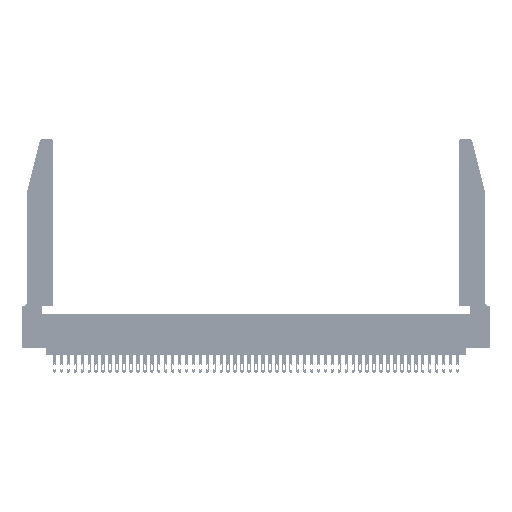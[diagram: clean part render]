
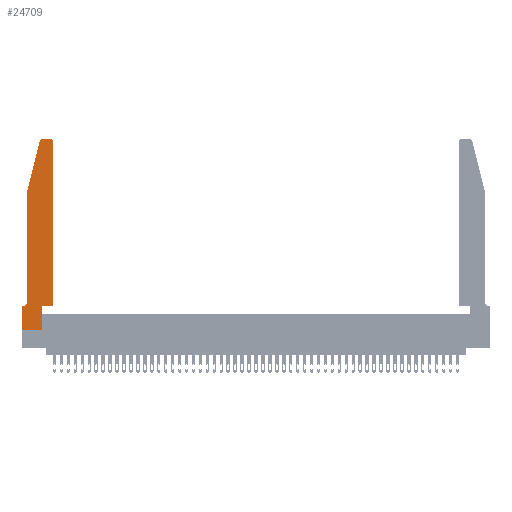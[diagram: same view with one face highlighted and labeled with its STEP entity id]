
A CAD part, top view. The second image highlights one B-rep face of the part: STEP entity #24709.
In plain terms, the highlighted planar face has unit normal (0, 0, 1).
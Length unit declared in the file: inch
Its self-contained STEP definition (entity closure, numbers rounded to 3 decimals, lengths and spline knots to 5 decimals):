
#183 = CIRCLE ( 'NONE', #768, 0.03 ) ;
#341 = DIRECTION ( 'NONE',  ( 0., 0., 1. ) ) ;
#351 = CARTESIAN_POINT ( 'NONE',  ( 0., 0.35, 0.37 ) ) ;
#488 = VECTOR ( 'NONE', #31601, 39.37008 ) ;
#573 = LINE ( 'NONE', #44899, #16606 ) ;
#768 = AXIS2_PLACEMENT_3D ( 'NONE', #4350, #11652, #34419 ) ;
#1428 = CARTESIAN_POINT ( 'NONE',  ( 0.2865, 0.35, 0.37 ) ) ;
#2223 = EDGE_CURVE ( 'NONE', #23543, #10127, #27594, .T. ) ;
#3217 = CARTESIAN_POINT ( 'NONE',  ( 0.2865, 0.35, 0.37 ) ) ;
#4350 = CARTESIAN_POINT ( 'NONE',  ( 0.4205, 2.72, 0.37 ) ) ;
#5069 = EDGE_CURVE ( 'NONE', #8838, #24708, #10907, .T. ) ;
#5454 = ORIENTED_EDGE ( 'NONE', *, *, #22700, .T. ) ;
#5991 = ORIENTED_EDGE ( 'NONE', *, *, #34411, .T. ) ;
#6038 = CARTESIAN_POINT ( 'NONE',  ( 0.4505, 0.35, 0.37 ) ) ;
#6975 = CARTESIAN_POINT ( 'NONE',  ( 0.4205, 2.75, 0.37 ) ) ;
#7641 = FACE_OUTER_BOUND ( 'NONE', #18019, .T. ) ;
#8130 = VERTEX_POINT ( 'NONE', #6975 ) ;
#8193 = LINE ( 'NONE', #1428, #44113 ) ;
#8483 = DIRECTION ( 'NONE',  ( -1., 0., 0. ) ) ;
#8838 = VERTEX_POINT ( 'NONE', #28938 ) ;
#9995 = DIRECTION ( 'NONE',  ( 1., 0., 0. ) ) ;
#10127 = VERTEX_POINT ( 'NONE', #24050 ) ;
#10395 = ORIENTED_EDGE ( 'NONE', *, *, #43474, .T. ) ;
#10548 = LINE ( 'NONE', #31767, #488 ) ;
#10907 = LINE ( 'NONE', #16419, #18087 ) ;
#10935 = ORIENTED_EDGE ( 'NONE', *, *, #39487, .T. ) ;
#10945 = VECTOR ( 'NONE', #14741, 39.37008 ) ;
#11652 = DIRECTION ( 'NONE',  ( 0., 0., 1. ) ) ;
#13085 = LINE ( 'NONE', #6038, #40780 ) ;
#13604 = AXIS2_PLACEMENT_3D ( 'NONE', #37990, #341, #46037 ) ;
#13871 = VERTEX_POINT ( 'NONE', #48773 ) ;
#14741 = DIRECTION ( 'NONE',  ( -1., 0., 0. ) ) ;
#14787 = EDGE_CURVE ( 'NONE', #31159, #8130, #183, .T. ) ;
#15461 = EDGE_CURVE ( 'NONE', #20353, #31159, #47329, .T. ) ;
#15609 = AXIS2_PLACEMENT_3D ( 'NONE', #18943, #45210, #19099 ) ;
#16419 = CARTESIAN_POINT ( 'NONE',  ( 0., 0., 0.37 ) ) ;
#16606 = VECTOR ( 'NONE', #29816, 39.37008 ) ;
#16960 = VERTEX_POINT ( 'NONE', #351 ) ;
#18019 = EDGE_LOOP ( 'NONE', ( #5991, #23481, #28074, #33410, #44886, #31744, #5454, #23098, #10395, #10935, #38307, #20407 ) ) ;
#18087 = VECTOR ( 'NONE', #31704, 39.37008 ) ;
#18943 = CARTESIAN_POINT ( 'NONE',  ( 0.284, 2.72, 0.37 ) ) ;
#19093 = CARTESIAN_POINT ( 'NONE',  ( 0.2865, 0., 0.37 ) ) ;
#19099 = DIRECTION ( 'NONE',  ( 1., 0., 0. ) ) ;
#19185 = VECTOR ( 'NONE', #32096, 39.37008 ) ;
#20084 = CARTESIAN_POINT ( 'NONE',  ( 0.0755, 2., 0.37 ) ) ;
#20353 = VERTEX_POINT ( 'NONE', #30305 ) ;
#20356 = LINE ( 'NONE', #20084, #19185 ) ;
#20407 = ORIENTED_EDGE ( 'NONE', *, *, #14787, .T. ) ;
#22700 = EDGE_CURVE ( 'NONE', #16960, #8838, #27076, .T. ) ;
#23098 = ORIENTED_EDGE ( 'NONE', *, *, #5069, .T. ) ;
#23361 = DIRECTION ( 'NONE',  ( 0., 0., -1. ) ) ;
#23481 = ORIENTED_EDGE ( 'NONE', *, *, #2223, .T. ) ;
#23543 = VERTEX_POINT ( 'NONE', #47120 ) ;
#23691 = CARTESIAN_POINT ( 'NONE',  ( 0.0055, 0.42, 0.37 ) ) ;
#24050 = CARTESIAN_POINT ( 'NONE',  ( 0.25487, 2.72718, 0.37 ) ) ;
#24708 = VERTEX_POINT ( 'NONE', #19093 ) ;
#24709 = ADVANCED_FACE ( 'NONE', ( #7641 ), #41604, .T. ) ;
#25517 = AXIS2_PLACEMENT_3D ( 'NONE', #23691, #23361, #8483 ) ;
#25555 = VERTEX_POINT ( 'NONE', #48331 ) ;
#25603 = VERTEX_POINT ( 'NONE', #26658 ) ;
#26585 = EDGE_CURVE ( 'NONE', #25603, #16960, #39849, .T. ) ;
#26658 = CARTESIAN_POINT ( 'NONE',  ( 0.0055, 0.35, 0.37 ) ) ;
#27047 = VERTEX_POINT ( 'NONE', #3217 ) ;
#27076 = LINE ( 'NONE', #34751, #48217 ) ;
#27254 = DIRECTION ( 'NONE',  ( 0., 1., 0. ) ) ;
#27514 = EDGE_CURVE ( 'NONE', #25555, #13871, #20356, .T. ) ;
#27594 = CIRCLE ( 'NONE', #15609, 0.03 ) ;
#28074 = ORIENTED_EDGE ( 'NONE', *, *, #37272, .T. ) ;
#28938 = CARTESIAN_POINT ( 'NONE',  ( 0., 0., 0.37 ) ) ;
#29816 = DIRECTION ( 'NONE',  ( -0.239, -0.971, 0. ) ) ;
#30305 = CARTESIAN_POINT ( 'NONE',  ( 0.4505, 0.35, 0.37 ) ) ;
#30716 = CIRCLE ( 'NONE', #25517, 0.07 ) ;
#31159 = VERTEX_POINT ( 'NONE', #36674 ) ;
#31601 = DIRECTION ( 'NONE',  ( -1., 0., 0. ) ) ;
#31704 = DIRECTION ( 'NONE',  ( 1., 0., 0. ) ) ;
#31744 = ORIENTED_EDGE ( 'NONE', *, *, #26585, .T. ) ;
#31767 = CARTESIAN_POINT ( 'NONE',  ( 0.2605, 2.75, 0.37 ) ) ;
#32096 = DIRECTION ( 'NONE',  ( 0., -1., 0. ) ) ;
#33410 = ORIENTED_EDGE ( 'NONE', *, *, #27514, .T. ) ;
#34261 = EDGE_CURVE ( 'NONE', #13871, #25603, #30716, .T. ) ;
#34411 = EDGE_CURVE ( 'NONE', #8130, #23543, #10548, .T. ) ;
#34419 = DIRECTION ( 'NONE',  ( 1., 0., 0. ) ) ;
#34751 = CARTESIAN_POINT ( 'NONE',  ( 0., 0., 0.37 ) ) ;
#36674 = CARTESIAN_POINT ( 'NONE',  ( 0.4505, 2.72, 0.37 ) ) ;
#37272 = EDGE_CURVE ( 'NONE', #10127, #25555, #573, .T. ) ;
#37598 = CARTESIAN_POINT ( 'NONE',  ( 0.0755, 0.35, 0.37 ) ) ;
#37990 = CARTESIAN_POINT ( 'NONE',  ( 0., 0.35, 0.37 ) ) ;
#38307 = ORIENTED_EDGE ( 'NONE', *, *, #15461, .T. ) ;
#38491 = DIRECTION ( 'NONE',  ( 0., -1., 0. ) ) ;
#39487 = EDGE_CURVE ( 'NONE', #27047, #20353, #13085, .T. ) ;
#39849 = LINE ( 'NONE', #37598, #10945 ) ;
#40780 = VECTOR ( 'NONE', #9995, 39.37008 ) ;
#41604 = PLANE ( 'NONE',  #13604 ) ;
#43474 = EDGE_CURVE ( 'NONE', #24708, #27047, #8193, .T. ) ;
#43698 = DIRECTION ( 'NONE',  ( 0., 1., 0. ) ) ;
#44113 = VECTOR ( 'NONE', #27254, 39.37008 ) ;
#44886 = ORIENTED_EDGE ( 'NONE', *, *, #34261, .T. ) ;
#44899 = CARTESIAN_POINT ( 'NONE',  ( 0.0755, 2., 0.37 ) ) ;
#45210 = DIRECTION ( 'NONE',  ( 0., 0., 1. ) ) ;
#46037 = DIRECTION ( 'NONE',  ( 1., 0., 0. ) ) ;
#46170 = VECTOR ( 'NONE', #43698, 39.37008 ) ;
#47120 = CARTESIAN_POINT ( 'NONE',  ( 0.284, 2.75, 0.37 ) ) ;
#47329 = LINE ( 'NONE', #47481, #46170 ) ;
#47481 = CARTESIAN_POINT ( 'NONE',  ( 0.4505, 0.35, 0.37 ) ) ;
#48217 = VECTOR ( 'NONE', #38491, 39.37008 ) ;
#48331 = CARTESIAN_POINT ( 'NONE',  ( 0.0755, 2., 0.37 ) ) ;
#48773 = CARTESIAN_POINT ( 'NONE',  ( 0.0755, 0.42, 0.37 ) ) ;
